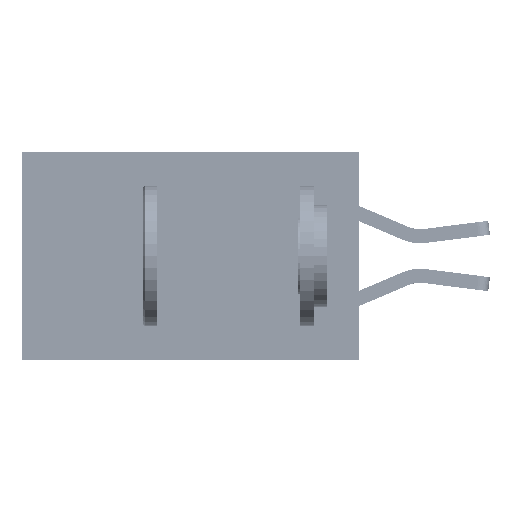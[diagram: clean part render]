
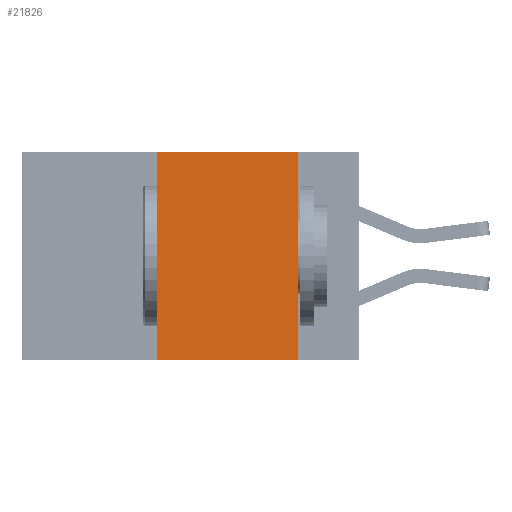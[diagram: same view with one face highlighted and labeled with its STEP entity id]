
A CAD part, left-side view. The second image highlights one B-rep face of the part: STEP entity #21826.
In plain terms, the highlighted planar face has unit normal (-1, 0, 0).
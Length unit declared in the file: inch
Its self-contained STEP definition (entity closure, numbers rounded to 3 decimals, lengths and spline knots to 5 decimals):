
#2540 = EDGE_LOOP ( 'NONE', ( #10566, #19836, #42570, #13616 ) ) ;
#4972 = EDGE_CURVE ( 'NONE', #42439, #28625, #36871, .T. ) ;
#5099 = CARTESIAN_POINT ( 'NONE',  ( 0., 0.6, 0. ) ) ;
#6284 = VECTOR ( 'NONE', #26712, 39.37008 ) ;
#7634 = CARTESIAN_POINT ( 'NONE',  ( 0., 0.11, 0. ) ) ;
#9234 = CARTESIAN_POINT ( 'NONE',  ( 0., 0.6, 0. ) ) ;
#10566 = ORIENTED_EDGE ( 'NONE', *, *, #10651, .F. ) ;
#10651 = EDGE_CURVE ( 'NONE', #28625, #16721, #35191, .T. ) ;
#10874 = DIRECTION ( 'NONE',  ( 0., 0., 1. ) ) ;
#13616 = ORIENTED_EDGE ( 'NONE', *, *, #32142, .T. ) ;
#16048 = VECTOR ( 'NONE', #38026, 39.37008 ) ;
#16721 = VERTEX_POINT ( 'NONE', #36141 ) ;
#18648 = CARTESIAN_POINT ( 'NONE',  ( 0., 0.36, 0. ) ) ;
#18851 = DIRECTION ( 'NONE',  ( 0., 0., -1. ) ) ;
#18897 = VECTOR ( 'NONE', #10874, 39.37008 ) ;
#19836 = ORIENTED_EDGE ( 'NONE', *, *, #4972, .F. ) ;
#20928 = CARTESIAN_POINT ( 'NONE',  ( 0., 0.36, 0. ) ) ;
#21826 = ADVANCED_FACE ( 'NONE', ( #44659 ), #39721, .F. ) ;
#24745 = CARTESIAN_POINT ( 'NONE',  ( 0., 0.36, -0.37 ) ) ;
#25786 = LINE ( 'NONE', #41993, #16048 ) ;
#26114 = DIRECTION ( 'NONE',  ( 1., 0., 0. ) ) ;
#26231 = AXIS2_PLACEMENT_3D ( 'NONE', #5099, #26114, #18851 ) ;
#26712 = DIRECTION ( 'NONE',  ( 0., -1., 0. ) ) ;
#28102 = LINE ( 'NONE', #20928, #18897 ) ;
#28251 = CARTESIAN_POINT ( 'NONE',  ( 0., 0.11, 0. ) ) ;
#28625 = VERTEX_POINT ( 'NONE', #28251 ) ;
#29120 = EDGE_CURVE ( 'NONE', #35009, #42439, #28102, .T. ) ;
#31967 = DIRECTION ( 'NONE',  ( 0., 0., -1. ) ) ;
#32142 = EDGE_CURVE ( 'NONE', #35009, #16721, #25786, .T. ) ;
#35009 = VERTEX_POINT ( 'NONE', #24745 ) ;
#35191 = LINE ( 'NONE', #7634, #38448 ) ;
#36141 = CARTESIAN_POINT ( 'NONE',  ( 0., 0.11, -0.37 ) ) ;
#36871 = LINE ( 'NONE', #9234, #6284 ) ;
#38026 = DIRECTION ( 'NONE',  ( 0., -1., 0. ) ) ;
#38448 = VECTOR ( 'NONE', #31967, 39.37008 ) ;
#39721 = PLANE ( 'NONE',  #26231 ) ;
#41993 = CARTESIAN_POINT ( 'NONE',  ( 0., 0.6, -0.37 ) ) ;
#42439 = VERTEX_POINT ( 'NONE', #18648 ) ;
#42570 = ORIENTED_EDGE ( 'NONE', *, *, #29120, .F. ) ;
#44659 = FACE_OUTER_BOUND ( 'NONE', #2540, .T. ) ;
